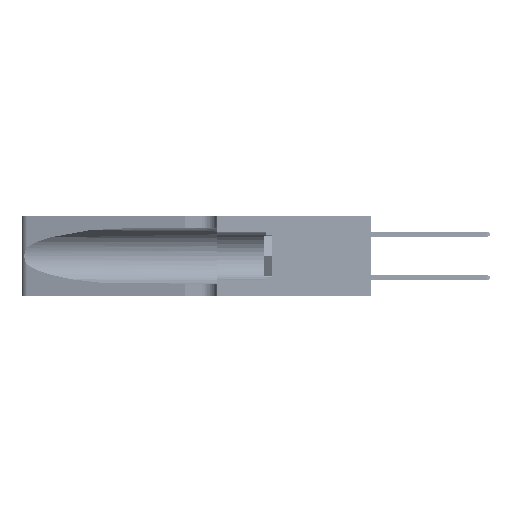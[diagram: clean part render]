
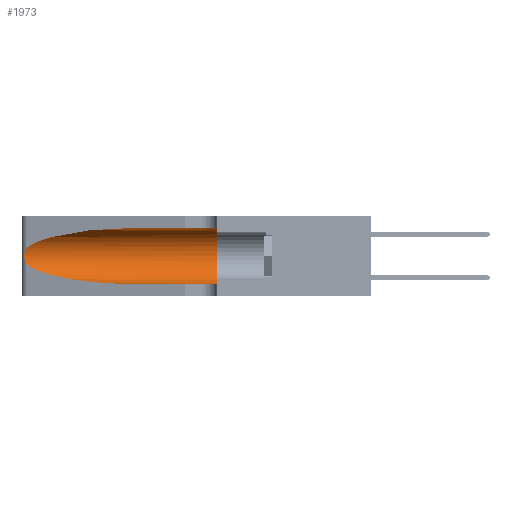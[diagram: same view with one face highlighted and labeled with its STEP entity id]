
A CAD part, left-side view. The second image highlights one B-rep face of the part: STEP entity #1973.
In plain terms, the highlighted cylindrical face has radius 3.308 mm (diameter 6.617 mm), a partial arc.
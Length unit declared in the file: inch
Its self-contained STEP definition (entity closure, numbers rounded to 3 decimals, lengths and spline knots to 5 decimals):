
#142 = CARTESIAN_POINT ( 'NONE',  ( 0.1305, 0.72297, 0.05475 ) ) ;
#690 = EDGE_CURVE ( 'NONE', #1405, #38491, #37468, .T. ) ;
#1405 = VERTEX_POINT ( 'NONE', #38710 ) ;
#1973 = ADVANCED_FACE ( 'NONE', ( #33963 ), #26134, .F. ) ;
#3261 = CARTESIAN_POINT ( 'NONE',  ( 0.25555, 1.22994, 0.2215 ) ) ;
#3301 = DIRECTION ( 'NONE',  ( 0., 0., -1. ) ) ;
#4257 = CARTESIAN_POINT ( 'NONE',  ( 0.1305, 1.61858, 0.05475 ) ) ;
#6514 = AXIS2_PLACEMENT_3D ( 'NONE', #35276, #46294, #12314 ) ;
#6658 = VERTEX_POINT ( 'NONE', #20737 ) ;
#6778 = CARTESIAN_POINT ( 'NONE',  ( 0.25487, 1.22718, 0.22369 ) ) ;
#6882 = EDGE_CURVE ( 'NONE', #6658, #39599, #47211, .T. ) ;
#8676 = CARTESIAN_POINT ( 'NONE',  ( 0.1305, 1.61858, 0.31525 ) ) ;
#10996 = CARTESIAN_POINT ( 'NONE',  ( 0.25487, 1.22718, 0.14631 ) ) ;
#11168 = CARTESIAN_POINT ( 'NONE',  ( 0.26075, 1.23896, 0.178 ) ) ;
#12287 = EDGE_CURVE ( 'NONE', #43096, #38491, #25520, .T. ) ;
#12314 = DIRECTION ( 'NONE',  ( 0., 0., 1. ) ) ;
#12906 = EDGE_CURVE ( 'NONE', #17077, #6658, #27900, .T. ) ;
#14928 = ORIENTED_EDGE ( 'NONE', *, *, #31672, .F. ) ;
#16298 = CARTESIAN_POINT ( 'NONE',  ( 0.25487, 1.22718, 0.22369 ) ) ;
#17077 = VERTEX_POINT ( 'NONE', #29219 ) ;
#18185 = CARTESIAN_POINT ( 'NONE',  ( 0.25789, 1.23486, 0.15765 ) ) ;
#18355 = CARTESIAN_POINT ( 'NONE',  ( 0.26018, 1.23835, 0.19895 ) ) ;
#18380 = LINE ( 'NONE', #8676, #26760 ) ;
#18394 = DIRECTION ( 'NONE',  ( 0., -1., 0. ) ) ;
#18862 = CARTESIAN_POINT ( 'NONE',  ( 0.25639, 1.23184, 0.21858 ) ) ;
#18993 =( BOUNDED_CURVE ( )  B_SPLINE_CURVE ( 3, ( #19072, #42510, #38340, #142 ),
 .UNSPECIFIED., .F., .T. ) 
 B_SPLINE_CURVE_WITH_KNOTS ( ( 4, 4 ),
 ( 3.44316, 4.71239 ),
 .UNSPECIFIED. ) 
 CURVE ( )  GEOMETRIC_REPRESENTATION_ITEM ( )  RATIONAL_B_SPLINE_CURVE ( ( 1., 0.87, 0.87, 1. ) ) 
 REPRESENTATION_ITEM ( '' )  );
#19064 = CARTESIAN_POINT ( 'NONE',  ( 0.1305, 1.61858, 0.185 ) ) ;
#19072 = CARTESIAN_POINT ( 'NONE',  ( 0.25487, 1.22718, 0.14631 ) ) ;
#19132 = ORIENTED_EDGE ( 'NONE', *, *, #22044, .T. ) ;
#19650 = CARTESIAN_POINT ( 'NONE',  ( 0.1305, 0.72297, 0.31525 ) ) ;
#20737 = CARTESIAN_POINT ( 'NONE',  ( 0.25487, 1.22718, 0.22369 ) ) ;
#20790 = ORIENTED_EDGE ( 'NONE', *, *, #690, .F. ) ;
#22044 = EDGE_CURVE ( 'NONE', #39599, #43096, #18993, .T. ) ;
#22231 = CARTESIAN_POINT ( 'NONE',  ( 0.25856, 1.23593, 0.16098 ) ) ;
#22396 = CARTESIAN_POINT ( 'NONE',  ( 0.25854, 1.2359, 0.20912 ) ) ;
#22565 = CARTESIAN_POINT ( 'NONE',  ( 0.25787, 1.23484, 0.2124 ) ) ;
#24272 = DIRECTION ( 'NONE',  ( 0., -1., 0. ) ) ;
#25520 = LINE ( 'NONE', #4257, #41083 ) ;
#26134 = CYLINDRICAL_SURFACE ( 'NONE', #47966, 0.13025 ) ;
#26760 = VECTOR ( 'NONE', #24272, 39.37008 ) ;
#26921 = DIRECTION ( 'NONE',  ( 0., -1., 0. ) ) ;
#27464 = CARTESIAN_POINT ( 'NONE',  ( 0.1305, 0.72297, 0.05475 ) ) ;
#27900 =( BOUNDED_CURVE ( )  B_SPLINE_CURVE ( 3, ( #19650, #35411, #42595, #16298 ),
 .UNSPECIFIED., .F., .F. ) 
 B_SPLINE_CURVE_WITH_KNOTS ( ( 4, 4 ),
 ( 1.5708, 2.84003 ),
 .UNSPECIFIED. ) 
 CURVE ( )  GEOMETRIC_REPRESENTATION_ITEM ( )  RATIONAL_B_SPLINE_CURVE ( ( 1., 0.87, 0.87, 1. ) ) 
 REPRESENTATION_ITEM ( '' )  );
#29219 = CARTESIAN_POINT ( 'NONE',  ( 0.1305, 0.72297, 0.31525 ) ) ;
#31672 = EDGE_CURVE ( 'NONE', #17077, #1405, #18380, .T. ) ;
#32726 = ORIENTED_EDGE ( 'NONE', *, *, #12287, .T. ) ;
#33963 = FACE_OUTER_BOUND ( 'NONE', #46685, .T. ) ;
#35276 = CARTESIAN_POINT ( 'NONE',  ( 0.1305, 0.35, 0.185 ) ) ;
#35411 = CARTESIAN_POINT ( 'NONE',  ( 0.18966, 0.96281, 0.31525 ) ) ;
#36728 = CARTESIAN_POINT ( 'NONE',  ( 0.25487, 1.22718, 0.14631 ) ) ;
#37468 = CIRCLE ( 'NONE', #6514, 0.13025 ) ;
#37962 = CARTESIAN_POINT ( 'NONE',  ( 0.26017, 1.23833, 0.17102 ) ) ;
#38340 = CARTESIAN_POINT ( 'NONE',  ( 0.18966, 0.96281, 0.05475 ) ) ;
#38491 = VERTEX_POINT ( 'NONE', #44876 ) ;
#38710 = CARTESIAN_POINT ( 'NONE',  ( 0.1305, 0.35, 0.31525 ) ) ;
#38861 = ORIENTED_EDGE ( 'NONE', *, *, #12906, .T. ) ;
#39599 = VERTEX_POINT ( 'NONE', #36728 ) ;
#40627 = ORIENTED_EDGE ( 'NONE', *, *, #6882, .T. ) ;
#41083 = VECTOR ( 'NONE', #26921, 39.37008 ) ;
#42510 = CARTESIAN_POINT ( 'NONE',  ( 0.2373, 1.15595, 0.08982 ) ) ;
#42595 = CARTESIAN_POINT ( 'NONE',  ( 0.2373, 1.15595, 0.28018 ) ) ;
#43096 = VERTEX_POINT ( 'NONE', #27464 ) ;
#44876 = CARTESIAN_POINT ( 'NONE',  ( 0.1305, 0.35, 0.05475 ) ) ;
#46294 = DIRECTION ( 'NONE',  ( 0., 1., 0. ) ) ;
#46685 = EDGE_LOOP ( 'NONE', ( #38861, #40627, #19132, #32726, #20790, #14928 ) ) ;
#47211 = B_SPLINE_CURVE_WITH_KNOTS ( 'NONE', 3,
 ( #6778, #3261, #18862, #22565, #22396, #18355, #49331, #11168, #37962, #22231, #18185, #49166, #48990, #10996 ),
 .UNSPECIFIED., .F., .F.,
 ( 4, 2, 2, 2, 2, 2, 4 ),
 ( 0., 0.00027, 0.00053, 0.00107, 0.0016, 0.00187, 0.00214 ),
 .UNSPECIFIED. ) ;
#47966 = AXIS2_PLACEMENT_3D ( 'NONE', #19064, #18394, #3301 ) ;
#48990 = CARTESIAN_POINT ( 'NONE',  ( 0.25555, 1.22993, 0.14849 ) ) ;
#49166 = CARTESIAN_POINT ( 'NONE',  ( 0.25639, 1.23186, 0.15144 ) ) ;
#49331 = CARTESIAN_POINT ( 'NONE',  ( 0.26075, 1.23896, 0.19203 ) ) ;
